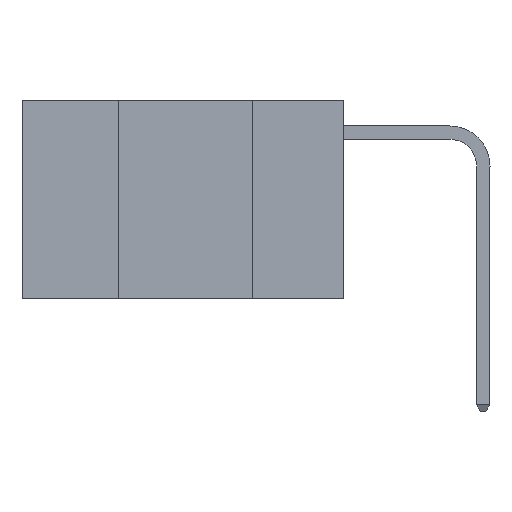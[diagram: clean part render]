
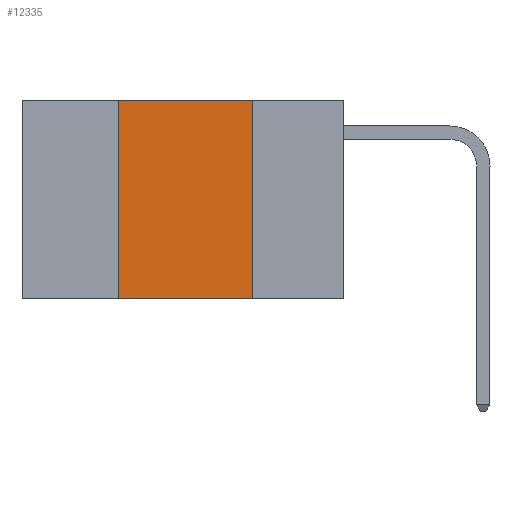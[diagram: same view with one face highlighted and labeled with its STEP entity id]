
A CAD part, left-side view. The second image highlights one B-rep face of the part: STEP entity #12335.
In plain terms, the highlighted planar face has unit normal (-1, 0, 0).
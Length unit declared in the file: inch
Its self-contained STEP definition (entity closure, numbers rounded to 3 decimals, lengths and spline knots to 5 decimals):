
#92 = EDGE_CURVE ( 'NONE', #8080, #9519, #18599, .T. ) ;
#1423 = DIRECTION ( 'NONE',  ( 1., 0., 0. ) ) ;
#1792 = AXIS2_PLACEMENT_3D ( 'NONE', #7145, #1423, #11525 ) ;
#2503 = ORIENTED_EDGE ( 'NONE', *, *, #12580, .T. ) ;
#2751 = VECTOR ( 'NONE', #12509, 39.37008 ) ;
#3105 = CARTESIAN_POINT ( 'NONE',  ( 0., 0.17, 0. ) ) ;
#3141 = CARTESIAN_POINT ( 'NONE',  ( 0., 0.42, 0. ) ) ;
#3168 = DIRECTION ( 'NONE',  ( 0., 0., -1. ) ) ;
#4413 = EDGE_LOOP ( 'NONE', ( #9271, #13105, #17464, #2503 ) ) ;
#4997 = LINE ( 'NONE', #3105, #16073 ) ;
#5761 = VERTEX_POINT ( 'NONE', #9898 ) ;
#7145 = CARTESIAN_POINT ( 'NONE',  ( 0., 0.6, 0. ) ) ;
#7707 = DIRECTION ( 'NONE',  ( 0., -1., 0. ) ) ;
#8080 = VERTEX_POINT ( 'NONE', #3141 ) ;
#8211 = CARTESIAN_POINT ( 'NONE',  ( 0., 0.6, 0. ) ) ;
#8931 = LINE ( 'NONE', #14950, #12317 ) ;
#9271 = ORIENTED_EDGE ( 'NONE', *, *, #9691, .F. ) ;
#9519 = VERTEX_POINT ( 'NONE', #15740 ) ;
#9691 = EDGE_CURVE ( 'NONE', #9519, #16411, #4997, .T. ) ;
#9898 = CARTESIAN_POINT ( 'NONE',  ( 0., 0.42, -0.37 ) ) ;
#10085 = PLANE ( 'NONE',  #1792 ) ;
#10318 = LINE ( 'NONE', #17741, #18505 ) ;
#10411 = DIRECTION ( 'NONE',  ( 0., 0., 1. ) ) ;
#11525 = DIRECTION ( 'NONE',  ( 0., 0., -1. ) ) ;
#11605 = EDGE_CURVE ( 'NONE', #5761, #8080, #10318, .T. ) ;
#12317 = VECTOR ( 'NONE', #7707, 39.37008 ) ;
#12335 = ADVANCED_FACE ( 'NONE', ( #12548 ), #10085, .F. ) ;
#12509 = DIRECTION ( 'NONE',  ( 0., -1., 0. ) ) ;
#12548 = FACE_OUTER_BOUND ( 'NONE', #4413, .T. ) ;
#12580 = EDGE_CURVE ( 'NONE', #5761, #16411, #8931, .T. ) ;
#13105 = ORIENTED_EDGE ( 'NONE', *, *, #92, .F. ) ;
#14950 = CARTESIAN_POINT ( 'NONE',  ( 0., 0.6, -0.37 ) ) ;
#15740 = CARTESIAN_POINT ( 'NONE',  ( 0., 0.17, 0. ) ) ;
#16073 = VECTOR ( 'NONE', #3168, 39.37008 ) ;
#16411 = VERTEX_POINT ( 'NONE', #17903 ) ;
#17464 = ORIENTED_EDGE ( 'NONE', *, *, #11605, .F. ) ;
#17741 = CARTESIAN_POINT ( 'NONE',  ( 0., 0.42, 0. ) ) ;
#17903 = CARTESIAN_POINT ( 'NONE',  ( 0., 0.17, -0.37 ) ) ;
#18505 = VECTOR ( 'NONE', #10411, 39.37008 ) ;
#18599 = LINE ( 'NONE', #8211, #2751 ) ;
